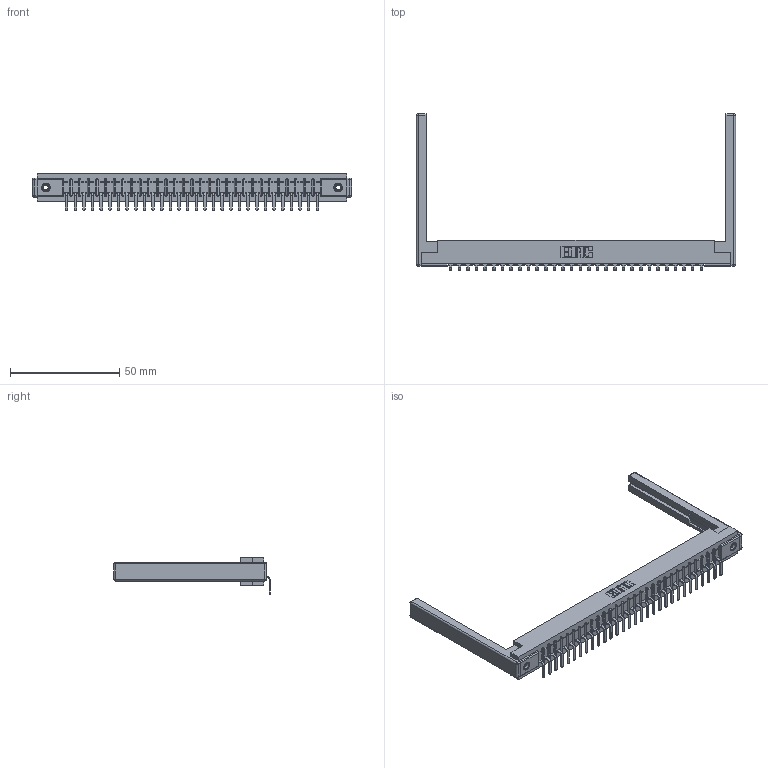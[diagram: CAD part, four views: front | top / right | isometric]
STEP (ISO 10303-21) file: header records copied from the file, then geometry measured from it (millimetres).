
FILE_DESCRIPTION (( 'STEP AP203' ), '1' );
FILE_NAME ('357-030-559-168.STEP', '2022-07-12T21:15:35', ( '' ), ( '' ), 'SwSTEP 2.0', 'SolidWorks 2020', '' );
FILE_SCHEMA (( 'CONFIG_CONTROL_DESIGN' ));
Length unit declared in the file: inch
Products named in the file (5): 345-250-001_345-250-001-102; 307 Part_.156 Dia Mounting Holes; 307-290-001_558 559 - 1 (Single); 307-220-068; 357-030-559-168
Assembly tree (35 placements, depth 2):
  357-030-559-168
    307 Part_.156 Dia Mounting Holes
    307-290-001_558 559 - 1 (Single)  x30
    307-220-068  x2
    345-250-001_345-250-001-102  x2
Bounding box: 146.3 x 71.67 x 16.8 mm (x, y, z)
Volume: 19527.9 mm3; surface area: 20039.5 mm2
Topology: 35 solids, 35 shells, 2103 faces, 5933 edges, 3810 vertices
Faces by surface type: plane 1328, cylinder 689, sphere 70, cone 12, torus 4
Entity records: 30061 total; most frequent: CARTESIAN_POINT 5025, ORIENTED_EDGE 5000, DIRECTION 4912, EDGE_CURVE 2500, LINE 1910, VECTOR 1910, VERTEX_POINT 1614, AXIS2_PLACEMENT_3D 1501
